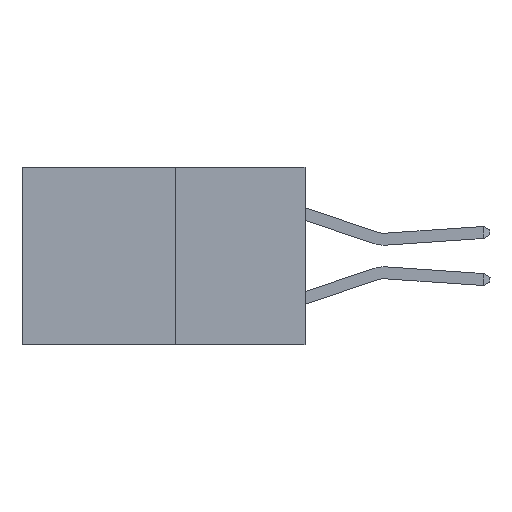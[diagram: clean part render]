
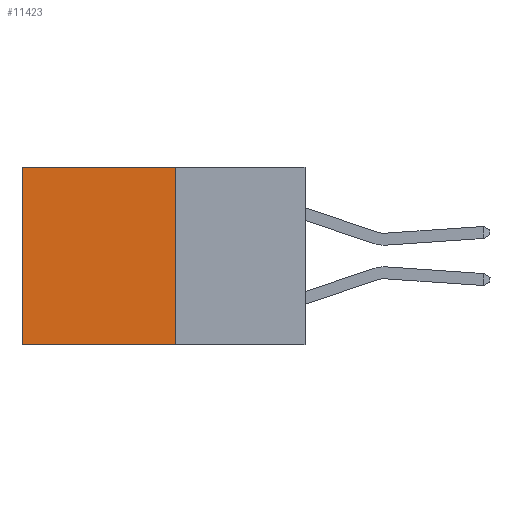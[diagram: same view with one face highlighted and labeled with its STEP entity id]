
A CAD part, left-side view. The second image highlights one B-rep face of the part: STEP entity #11423.
In plain terms, the highlighted planar face has unit normal (-1, 0, 0).
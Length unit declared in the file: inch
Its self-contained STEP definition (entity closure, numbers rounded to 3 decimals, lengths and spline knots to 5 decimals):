
#102 = VECTOR ( 'NONE', #430, 39.37008 ) ;
#430 = DIRECTION ( 'NONE',  ( 0., 1., 0. ) ) ;
#652 = LINE ( 'NONE', #18196, #102 ) ;
#1083 = LINE ( 'NONE', #17432, #18921 ) ;
#1139 = EDGE_LOOP ( 'NONE', ( #1190, #14669, #20445, #1512 ) ) ;
#1190 = ORIENTED_EDGE ( 'NONE', *, *, #4304, .T. ) ;
#1512 = ORIENTED_EDGE ( 'NONE', *, *, #12235, .T. ) ;
#1529 = LINE ( 'NONE', #10604, #19908 ) ;
#1533 = VERTEX_POINT ( 'NONE', #14768 ) ;
#4304 = EDGE_CURVE ( 'NONE', #1533, #7008, #10913, .T. ) ;
#5231 = CARTESIAN_POINT ( 'NONE',  ( 0.277, 0.27, -0.37 ) ) ;
#6201 = VECTOR ( 'NONE', #19433, 39.37008 ) ;
#7008 = VERTEX_POINT ( 'NONE', #22600 ) ;
#7264 = FACE_OUTER_BOUND ( 'NONE', #1139, .T. ) ;
#8020 = EDGE_CURVE ( 'NONE', #16974, #19970, #1529, .T. ) ;
#8410 = CARTESIAN_POINT ( 'NONE',  ( 0.277, 0.27, -0.37 ) ) ;
#8740 = PLANE ( 'NONE',  #9082 ) ;
#9082 = AXIS2_PLACEMENT_3D ( 'NONE', #5231, #21222, #10582 ) ;
#10525 = DIRECTION ( 'NONE',  ( 0., 0., -1. ) ) ;
#10582 = DIRECTION ( 'NONE',  ( 0., 0., -1. ) ) ;
#10604 = CARTESIAN_POINT ( 'NONE',  ( 0.277, 0.27, -0.37 ) ) ;
#10913 = LINE ( 'NONE', #19404, #6201 ) ;
#11423 = ADVANCED_FACE ( 'NONE', ( #7264 ), #8740, .F. ) ;
#12235 = EDGE_CURVE ( 'NONE', #16974, #1533, #1083, .T. ) ;
#14669 = ORIENTED_EDGE ( 'NONE', *, *, #15878, .F. ) ;
#14768 = CARTESIAN_POINT ( 'NONE',  ( 0.277, 0.59, 0. ) ) ;
#15878 = EDGE_CURVE ( 'NONE', #19970, #7008, #652, .T. ) ;
#16974 = VERTEX_POINT ( 'NONE', #21109 ) ;
#17432 = CARTESIAN_POINT ( 'NONE',  ( 0.277, 0.27, 0. ) ) ;
#18196 = CARTESIAN_POINT ( 'NONE',  ( 0.277, 0.27, -0.37 ) ) ;
#18921 = VECTOR ( 'NONE', #19194, 39.37008 ) ;
#19194 = DIRECTION ( 'NONE',  ( 0., 1., 0. ) ) ;
#19404 = CARTESIAN_POINT ( 'NONE',  ( 0.277, 0.59, -0.37 ) ) ;
#19433 = DIRECTION ( 'NONE',  ( 0., 0., -1. ) ) ;
#19908 = VECTOR ( 'NONE', #10525, 39.37008 ) ;
#19970 = VERTEX_POINT ( 'NONE', #8410 ) ;
#20445 = ORIENTED_EDGE ( 'NONE', *, *, #8020, .F. ) ;
#21109 = CARTESIAN_POINT ( 'NONE',  ( 0.277, 0.27, 0. ) ) ;
#21222 = DIRECTION ( 'NONE',  ( 1., 0., 0. ) ) ;
#22600 = CARTESIAN_POINT ( 'NONE',  ( 0.277, 0.59, -0.37 ) ) ;
